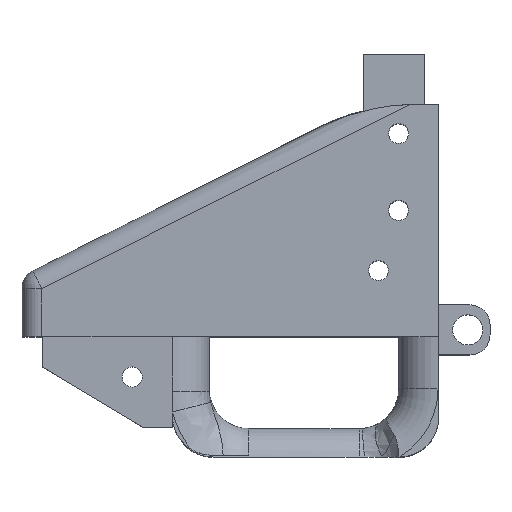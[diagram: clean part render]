
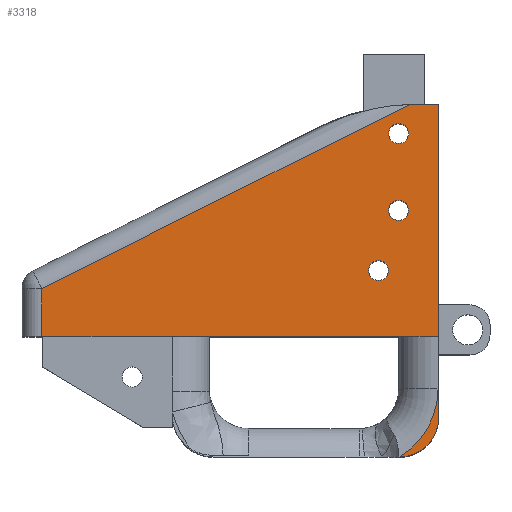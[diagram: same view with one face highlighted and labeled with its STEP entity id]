
A CAD part, top view. The second image highlights one B-rep face of the part: STEP entity #3318.
In plain terms, the highlighted planar face has unit normal (0, 0, 1).
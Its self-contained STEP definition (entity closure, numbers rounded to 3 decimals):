
#44 = EDGE_CURVE ( 'NONE', #4464, #919, #1198, .T. ) ;
#155 = CARTESIAN_POINT ( 'NONE',  ( -92.837, 0., 69.85 ) ) ;
#231 = DIRECTION ( 'NONE',  ( 1., 0., 0. ) ) ;
#291 = EDGE_LOOP ( 'NONE', ( #1063, #4684, #3095, #2968, #5459, #635, #1682, #3552, #4190, #5456, #3773 ) ) ;
#342 = EDGE_CURVE ( 'NONE', #860, #704, #4645, .T. ) ;
#389 = CIRCLE ( 'NONE', #1953, 2.54 ) ;
#392 = VECTOR ( 'NONE', #570, 1000. ) ;
#413 = EDGE_LOOP ( 'NONE', ( #4662, #2105 ) ) ;
#427 = DIRECTION ( 'NONE',  ( 1., 0., 0. ) ) ;
#467 = VERTEX_POINT ( 'NONE', #5259 ) ;
#561 = EDGE_CURVE ( 'NONE', #3544, #1950, #4360, .T. ) ;
#570 = DIRECTION ( 'NONE',  ( 0., 1., 0. ) ) ;
#635 = ORIENTED_EDGE ( 'NONE', *, *, #1783, .T. ) ;
#665 = CARTESIAN_POINT ( 'NONE',  ( -125.937, 0., 69.85 ) ) ;
#691 = EDGE_CURVE ( 'NONE', #4296, #3544, #3374, .T. ) ;
#704 = VERTEX_POINT ( 'NONE', #4854 ) ;
#759 = EDGE_CURVE ( 'NONE', #5796, #1480, #4146, .T. ) ;
#819 = CARTESIAN_POINT ( 'NONE',  ( -25.4, -30.48, 69.85 ) ) ;
#833 = DIRECTION ( 'NONE',  ( 1., 0., 0. ) ) ;
#849 = DIRECTION ( 'NONE',  ( 1., 0., 0. ) ) ;
#850 = CARTESIAN_POINT ( 'NONE',  ( -33.02, 32.004, 69.85 ) ) ;
#860 = VERTEX_POINT ( 'NONE', #5310 ) ;
#869 = DIRECTION ( 'NONE',  ( 0., 0., -1. ) ) ;
#871 = VERTEX_POINT ( 'NONE', #5777 ) ;
#919 = VERTEX_POINT ( 'NONE', #3066 ) ;
#978 = CARTESIAN_POINT ( 'NONE',  ( -35.56, -30.48, 69.85 ) ) ;
#1003 = DIRECTION ( 'NONE',  ( 1., 0., 0. ) ) ;
#1063 = ORIENTED_EDGE ( 'NONE', *, *, #2166, .T. ) ;
#1068 = DIRECTION ( 'NONE',  ( 0., 0., 1. ) ) ;
#1098 = CARTESIAN_POINT ( 'NONE',  ( -25.56, -13.241, 69.85 ) ) ;
#1111 = EDGE_CURVE ( 'NONE', #1950, #871, #1797, .T. ) ;
#1117 = CIRCLE ( 'NONE', #4079, 2.54 ) ;
#1142 = VERTEX_POINT ( 'NONE', #1491 ) ;
#1198 = CIRCLE ( 'NONE', #1382, 2.54 ) ;
#1206 = DIRECTION ( 'NONE',  ( 1., 0., 0. ) ) ;
#1249 = FACE_BOUND ( 'NONE', #4467, .T. ) ;
#1254 = LINE ( 'NONE', #3809, #4209 ) ;
#1288 = DIRECTION ( 'NONE',  ( 1., 0., 0. ) ) ;
#1307 = CARTESIAN_POINT ( 'NONE',  ( -35.4, -20.48, 69.85 ) ) ;
#1346 = DIRECTION ( 'NONE',  ( 0., 0., 1. ) ) ;
#1382 = AXIS2_PLACEMENT_3D ( 'NONE', #2624, #4416, #1288 ) ;
#1395 = DIRECTION ( 'NONE',  ( 1., 0., 0. ) ) ;
#1474 = CARTESIAN_POINT ( 'NONE',  ( -33.02, 51.46, 69.85 ) ) ;
#1480 = VERTEX_POINT ( 'NONE', #1848 ) ;
#1491 = CARTESIAN_POINT ( 'NONE',  ( -125.937, 12.154, 69.85 ) ) ;
#1576 = DIRECTION ( 'NONE',  ( 1., 0., 0. ) ) ;
#1588 = EDGE_CURVE ( 'NONE', #3100, #3266, #4347, .T. ) ;
#1605 = AXIS2_PLACEMENT_3D ( 'NONE', #3113, #869, #1395 ) ;
#1642 = DIRECTION ( 'NONE',  ( -0.894, -0.448, 0. ) ) ;
#1682 = ORIENTED_EDGE ( 'NONE', *, *, #342, .T. ) ;
#1710 = CARTESIAN_POINT ( 'NONE',  ( -35.56, 32.004, 69.85 ) ) ;
#1783 = EDGE_CURVE ( 'NONE', #5251, #860, #2291, .T. ) ;
#1797 = CIRCLE ( 'NONE', #1903, 55.773 ) ;
#1821 = CARTESIAN_POINT ( 'NONE',  ( -25.4, 58.826, 69.85 ) ) ;
#1848 = CARTESIAN_POINT ( 'NONE',  ( -38.1, 51.46, 69.85 ) ) ;
#1903 = AXIS2_PLACEMENT_3D ( 'NONE', #4625, #4194, #3712 ) ;
#1943 = AXIS2_PLACEMENT_3D ( 'NONE', #5117, #1068, #1576 ) ;
#1945 = VECTOR ( 'NONE', #849, 1000. ) ;
#1950 = VERTEX_POINT ( 'NONE', #4178 ) ;
#1953 = AXIS2_PLACEMENT_3D ( 'NONE', #4454, #2634, #833 ) ;
#2011 = CARTESIAN_POINT ( 'NONE',  ( -25.4, 58.826, 69.85 ) ) ;
#2063 = CARTESIAN_POINT ( 'NONE',  ( -35.56, 32.004, 69.85 ) ) ;
#2090 = VECTOR ( 'NONE', #4994, 1000. ) ;
#2105 = ORIENTED_EDGE ( 'NONE', *, *, #44, .F. ) ;
#2156 = DIRECTION ( 'NONE',  ( 0., 0., 1. ) ) ;
#2166 = EDGE_CURVE ( 'NONE', #871, #1142, #1254, .T. ) ;
#2269 = EDGE_CURVE ( 'NONE', #5530, #5239, #4841, .T. ) ;
#2291 = CIRCLE ( 'NONE', #1605, 20. ) ;
#2297 = FACE_BOUND ( 'NONE', #5329, .T. ) ;
#2400 = EDGE_CURVE ( 'NONE', #1480, #5796, #389, .T. ) ;
#2498 = CARTESIAN_POINT ( 'NONE',  ( -35.56, 51.46, 69.85 ) ) ;
#2516 = AXIS2_PLACEMENT_3D ( 'NONE', #2063, #3415, #3923 ) ;
#2518 = CIRCLE ( 'NONE', #2985, 2.54 ) ;
#2554 = CARTESIAN_POINT ( 'NONE',  ( -130.937, 0., 69.85 ) ) ;
#2581 = CARTESIAN_POINT ( 'NONE',  ( -40.64, 16.764, 69.85 ) ) ;
#2624 = CARTESIAN_POINT ( 'NONE',  ( -40.64, 16.764, 69.85 ) ) ;
#2634 = DIRECTION ( 'NONE',  ( 0., 0., 1. ) ) ;
#2806 = LINE ( 'NONE', #665, #5720 ) ;
#2936 = VECTOR ( 'NONE', #3759, 1000. ) ;
#2968 = ORIENTED_EDGE ( 'NONE', *, *, #5395, .T. ) ;
#2985 = AXIS2_PLACEMENT_3D ( 'NONE', #1710, #2156, #231 ) ;
#2990 = EDGE_CURVE ( 'NONE', #704, #4296, #4231, .T. ) ;
#3064 = AXIS2_PLACEMENT_3D ( 'NONE', #1307, #1346, #427 ) ;
#3066 = CARTESIAN_POINT ( 'NONE',  ( -43.18, 16.764, 69.85 ) ) ;
#3095 = ORIENTED_EDGE ( 'NONE', *, *, #2269, .T. ) ;
#3100 = VERTEX_POINT ( 'NONE', #850 ) ;
#3113 = CARTESIAN_POINT ( 'NONE',  ( -45.56, -13.241, 69.85 ) ) ;
#3132 = FACE_BOUND ( 'NONE', #413, .T. ) ;
#3266 = VERTEX_POINT ( 'NONE', #3338 ) ;
#3295 = CARTESIAN_POINT ( 'NONE',  ( -25.56, 3.077, 69.85 ) ) ;
#3318 = ADVANCED_FACE ( 'NONE', ( #3363, #1249, #2297, #3132 ), #4646, .T. ) ;
#3338 = CARTESIAN_POINT ( 'NONE',  ( -38.1, 32.004, 69.85 ) ) ;
#3363 = FACE_OUTER_BOUND ( 'NONE', #291, .T. ) ;
#3374 = LINE ( 'NONE', #819, #392 ) ;
#3415 = DIRECTION ( 'NONE',  ( 0., 0., 1. ) ) ;
#3544 = VERTEX_POINT ( 'NONE', #2011 ) ;
#3552 = ORIENTED_EDGE ( 'NONE', *, *, #2990, .T. ) ;
#3705 = DIRECTION ( 'NONE',  ( 1., 0., 0. ) ) ;
#3712 = DIRECTION ( 'NONE',  ( 1., 0., 0. ) ) ;
#3759 = DIRECTION ( 'NONE',  ( 0., -1., 0. ) ) ;
#3763 = CARTESIAN_POINT ( 'NONE',  ( -25.4, -20.48, 69.85 ) ) ;
#3773 = ORIENTED_EDGE ( 'NONE', *, *, #1111, .T. ) ;
#3809 = CARTESIAN_POINT ( 'NONE',  ( -128.696, 10.77, 69.85 ) ) ;
#3923 = DIRECTION ( 'NONE',  ( 1., 0., 0. ) ) ;
#3951 = DIRECTION ( 'NONE',  ( 0., 0., 1. ) ) ;
#3986 = CARTESIAN_POINT ( 'NONE',  ( -130.937, 0., 69.85 ) ) ;
#4079 = AXIS2_PLACEMENT_3D ( 'NONE', #2581, #3951, #3705 ) ;
#4094 = ORIENTED_EDGE ( 'NONE', *, *, #2400, .F. ) ;
#4146 = CIRCLE ( 'NONE', #4370, 2.54 ) ;
#4178 = CARTESIAN_POINT ( 'NONE',  ( -32.37, 58.826, 69.85 ) ) ;
#4190 = ORIENTED_EDGE ( 'NONE', *, *, #691, .T. ) ;
#4194 = DIRECTION ( 'NONE',  ( 0., 0., 1. ) ) ;
#4209 = VECTOR ( 'NONE', #1642, 1000. ) ;
#4224 = VECTOR ( 'NONE', #1003, 1000. ) ;
#4231 = CIRCLE ( 'NONE', #3064, 10. ) ;
#4296 = VERTEX_POINT ( 'NONE', #3763 ) ;
#4317 = ORIENTED_EDGE ( 'NONE', *, *, #1588, .F. ) ;
#4336 = DIRECTION ( 'NONE',  ( 1., 0., 0. ) ) ;
#4347 = CIRCLE ( 'NONE', #2516, 2.54 ) ;
#4360 = LINE ( 'NONE', #1821, #2090 ) ;
#4370 = AXIS2_PLACEMENT_3D ( 'NONE', #2498, #5672, #1206 ) ;
#4416 = DIRECTION ( 'NONE',  ( 0., 0., 1. ) ) ;
#4427 = LINE ( 'NONE', #3295, #2936 ) ;
#4454 = CARTESIAN_POINT ( 'NONE',  ( -35.56, 51.46, 69.85 ) ) ;
#4464 = VERTEX_POINT ( 'NONE', #5232 ) ;
#4467 = EDGE_LOOP ( 'NONE', ( #5374, #4317 ) ) ;
#4525 = ORIENTED_EDGE ( 'NONE', *, *, #759, .F. ) ;
#4625 = CARTESIAN_POINT ( 'NONE',  ( -30.767, 3.077, 69.85 ) ) ;
#4639 = LINE ( 'NONE', #3986, #1945 ) ;
#4645 = LINE ( 'NONE', #978, #4224 ) ;
#4646 = PLANE ( 'NONE',  #1943 ) ;
#4662 = ORIENTED_EDGE ( 'NONE', *, *, #5687, .F. ) ;
#4684 = ORIENTED_EDGE ( 'NONE', *, *, #4771, .T. ) ;
#4771 = EDGE_CURVE ( 'NONE', #1142, #5530, #2806, .T. ) ;
#4841 = LINE ( 'NONE', #2554, #5064 ) ;
#4854 = CARTESIAN_POINT ( 'NONE',  ( -35.4, -30.48, 69.85 ) ) ;
#4936 = CARTESIAN_POINT ( 'NONE',  ( -125.937, 0., 69.85 ) ) ;
#4994 = DIRECTION ( 'NONE',  ( -1., 0., 0. ) ) ;
#5064 = VECTOR ( 'NONE', #4336, 1000. ) ;
#5117 = CARTESIAN_POINT ( 'NONE',  ( -30.767, 3.077, 69.85 ) ) ;
#5164 = DIRECTION ( 'NONE',  ( 0., -1., 0. ) ) ;
#5232 = CARTESIAN_POINT ( 'NONE',  ( -38.1, 16.764, 69.85 ) ) ;
#5239 = VERTEX_POINT ( 'NONE', #155 ) ;
#5251 = VERTEX_POINT ( 'NONE', #1098 ) ;
#5259 = CARTESIAN_POINT ( 'NONE',  ( -25.56, 0., 69.85 ) ) ;
#5310 = CARTESIAN_POINT ( 'NONE',  ( -35.42, -30.48, 69.85 ) ) ;
#5327 = EDGE_CURVE ( 'NONE', #3266, #3100, #2518, .T. ) ;
#5329 = EDGE_LOOP ( 'NONE', ( #4094, #4525 ) ) ;
#5374 = ORIENTED_EDGE ( 'NONE', *, *, #5327, .F. ) ;
#5395 = EDGE_CURVE ( 'NONE', #5239, #467, #4639, .T. ) ;
#5456 = ORIENTED_EDGE ( 'NONE', *, *, #561, .T. ) ;
#5459 = ORIENTED_EDGE ( 'NONE', *, *, #5813, .T. ) ;
#5530 = VERTEX_POINT ( 'NONE', #4936 ) ;
#5672 = DIRECTION ( 'NONE',  ( 0., 0., 1. ) ) ;
#5687 = EDGE_CURVE ( 'NONE', #919, #4464, #1117, .T. ) ;
#5720 = VECTOR ( 'NONE', #5164, 1000. ) ;
#5777 = CARTESIAN_POINT ( 'NONE',  ( -32.879, 58.809, 69.85 ) ) ;
#5796 = VERTEX_POINT ( 'NONE', #1474 ) ;
#5813 = EDGE_CURVE ( 'NONE', #467, #5251, #4427, .T. ) ;
